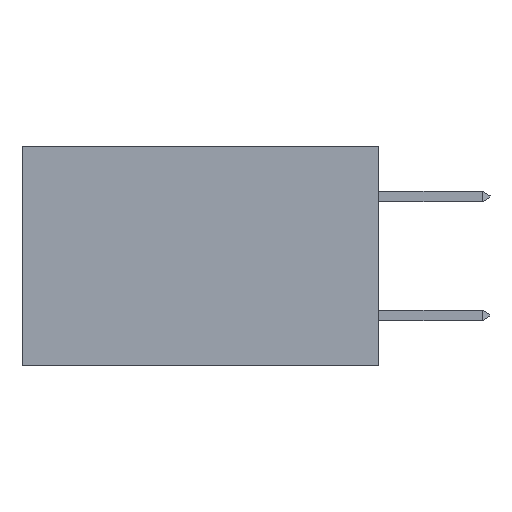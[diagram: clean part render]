
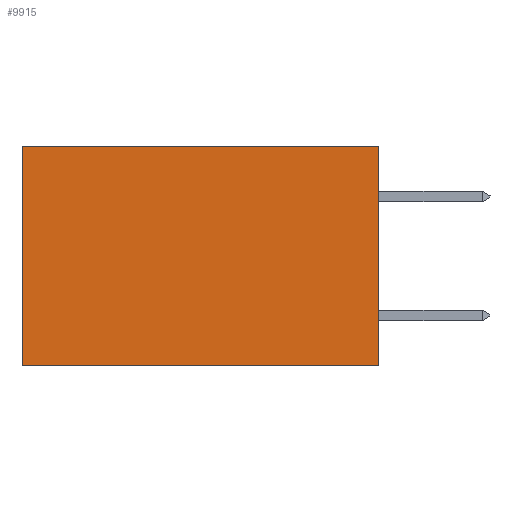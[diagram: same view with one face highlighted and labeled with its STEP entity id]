
A CAD part, left-side view. The second image highlights one B-rep face of the part: STEP entity #9915.
In plain terms, the highlighted planar face has unit normal (-1, 0, 0).
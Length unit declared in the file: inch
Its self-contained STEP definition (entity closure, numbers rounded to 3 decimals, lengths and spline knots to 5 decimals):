
#192 = CARTESIAN_POINT ( 'NONE',  ( 0.2615, 0., 0. ) ) ;
#1121 = VERTEX_POINT ( 'NONE', #11900 ) ;
#1265 = AXIS2_PLACEMENT_3D ( 'NONE', #11468, #5885, #12625 ) ;
#1281 = ORIENTED_EDGE ( 'NONE', *, *, #2695, .F. ) ;
#1701 = LINE ( 'NONE', #7863, #7505 ) ;
#2198 = EDGE_LOOP ( 'NONE', ( #10578, #10490, #1281, #11506 ) ) ;
#2277 = CARTESIAN_POINT ( 'NONE',  ( 0.2615, 0., -0.37 ) ) ;
#2470 = CARTESIAN_POINT ( 'NONE',  ( 0.2615, 0.6, -0.37 ) ) ;
#2695 = EDGE_CURVE ( 'NONE', #1121, #8715, #12650, .T. ) ;
#3339 = VECTOR ( 'NONE', #9191, 39.37008 ) ;
#3554 = CARTESIAN_POINT ( 'NONE',  ( 0.2615, 0.6, -0.37 ) ) ;
#3938 = VECTOR ( 'NONE', #7916, 39.37008 ) ;
#4525 = CARTESIAN_POINT ( 'NONE',  ( 0.2615, 0., -0.37 ) ) ;
#5825 = LINE ( 'NONE', #3554, #3339 ) ;
#5874 = EDGE_CURVE ( 'NONE', #6539, #13081, #5825, .T. ) ;
#5885 = DIRECTION ( 'NONE',  ( 1., 0., 0. ) ) ;
#5983 = LINE ( 'NONE', #192, #3938 ) ;
#5991 = DIRECTION ( 'NONE',  ( 0., 0., -1. ) ) ;
#6058 = EDGE_CURVE ( 'NONE', #8715, #13081, #1701, .T. ) ;
#6539 = VERTEX_POINT ( 'NONE', #13867 ) ;
#7505 = VECTOR ( 'NONE', #8929, 39.37008 ) ;
#7863 = CARTESIAN_POINT ( 'NONE',  ( 0.2615, 0., -0.37 ) ) ;
#7916 = DIRECTION ( 'NONE',  ( 0., 1., 0. ) ) ;
#8104 = FACE_OUTER_BOUND ( 'NONE', #2198, .T. ) ;
#8715 = VERTEX_POINT ( 'NONE', #4525 ) ;
#8929 = DIRECTION ( 'NONE',  ( 0., 1., 0. ) ) ;
#9191 = DIRECTION ( 'NONE',  ( 0., 0., -1. ) ) ;
#9530 = EDGE_CURVE ( 'NONE', #1121, #6539, #5983, .T. ) ;
#9915 = ADVANCED_FACE ( 'NONE', ( #8104 ), #13759, .F. ) ;
#10299 = VECTOR ( 'NONE', #5991, 39.37008 ) ;
#10490 = ORIENTED_EDGE ( 'NONE', *, *, #6058, .F. ) ;
#10578 = ORIENTED_EDGE ( 'NONE', *, *, #5874, .T. ) ;
#11468 = CARTESIAN_POINT ( 'NONE',  ( 0.2615, 0., -0.37 ) ) ;
#11506 = ORIENTED_EDGE ( 'NONE', *, *, #9530, .T. ) ;
#11900 = CARTESIAN_POINT ( 'NONE',  ( 0.2615, 0., 0. ) ) ;
#12625 = DIRECTION ( 'NONE',  ( 0., 0., -1. ) ) ;
#12650 = LINE ( 'NONE', #2277, #10299 ) ;
#13081 = VERTEX_POINT ( 'NONE', #2470 ) ;
#13759 = PLANE ( 'NONE',  #1265 ) ;
#13867 = CARTESIAN_POINT ( 'NONE',  ( 0.2615, 0.6, 0. ) ) ;
